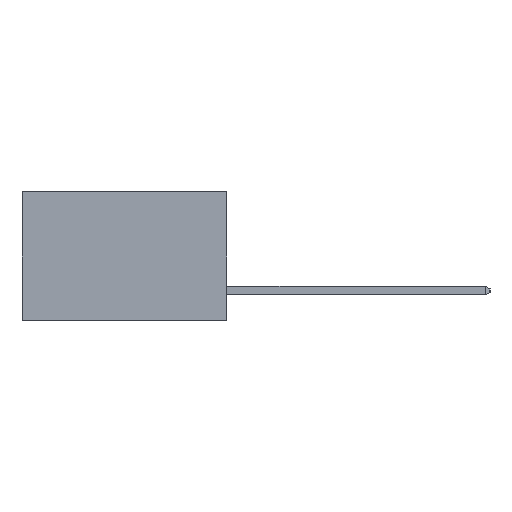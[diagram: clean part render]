
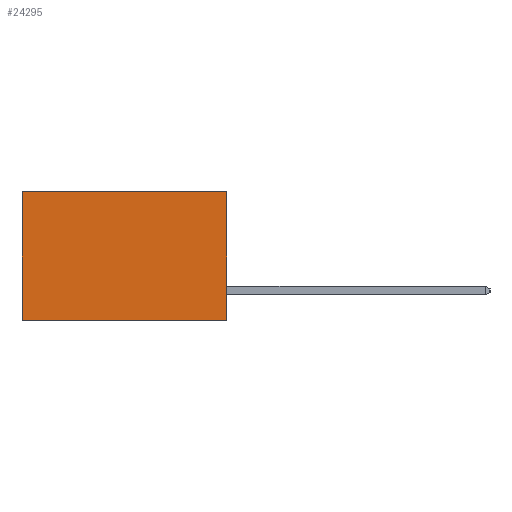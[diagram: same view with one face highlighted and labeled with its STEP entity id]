
A CAD part, left-side view. The second image highlights one B-rep face of the part: STEP entity #24295.
In plain terms, the highlighted planar face has unit normal (-1, 0, 0).
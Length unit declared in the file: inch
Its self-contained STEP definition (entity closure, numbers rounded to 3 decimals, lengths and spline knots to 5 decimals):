
#108 = FACE_OUTER_BOUND ( 'NONE', #27243, .T. ) ;
#1035 = CARTESIAN_POINT ( 'NONE',  ( 0.277, 0., -0.37 ) ) ;
#3607 = VERTEX_POINT ( 'NONE', #18103 ) ;
#3843 = VERTEX_POINT ( 'NONE', #1035 ) ;
#4120 = ORIENTED_EDGE ( 'NONE', *, *, #9924, .T. ) ;
#5090 = DIRECTION ( 'NONE',  ( 1., 0., 0. ) ) ;
#5503 = EDGE_CURVE ( 'NONE', #3607, #3843, #12586, .T. ) ;
#6590 = CARTESIAN_POINT ( 'NONE',  ( 0.277, 0.59, -0.37 ) ) ;
#7765 = CARTESIAN_POINT ( 'NONE',  ( 0.277, 0.59, 0. ) ) ;
#8504 = VERTEX_POINT ( 'NONE', #24318 ) ;
#8766 = CARTESIAN_POINT ( 'NONE',  ( 0.277, 0., -0.37 ) ) ;
#9924 = EDGE_CURVE ( 'NONE', #3607, #28241, #12692, .T. ) ;
#10095 = ORIENTED_EDGE ( 'NONE', *, *, #5503, .F. ) ;
#11259 = LINE ( 'NONE', #6590, #22120 ) ;
#11302 = DIRECTION ( 'NONE',  ( 0., 1., 0. ) ) ;
#11769 = PLANE ( 'NONE',  #25907 ) ;
#12586 = LINE ( 'NONE', #17600, #17746 ) ;
#12692 = LINE ( 'NONE', #15643, #17858 ) ;
#13662 = ORIENTED_EDGE ( 'NONE', *, *, #13940, .F. ) ;
#13713 = VECTOR ( 'NONE', #17547, 39.37008 ) ;
#13940 = EDGE_CURVE ( 'NONE', #3843, #8504, #18876, .T. ) ;
#15643 = CARTESIAN_POINT ( 'NONE',  ( 0.277, 0., 0. ) ) ;
#16268 = ORIENTED_EDGE ( 'NONE', *, *, #20449, .T. ) ;
#17547 = DIRECTION ( 'NONE',  ( 0., 1., 0. ) ) ;
#17600 = CARTESIAN_POINT ( 'NONE',  ( 0.277, 0., -0.37 ) ) ;
#17665 = DIRECTION ( 'NONE',  ( 0., 0., -1. ) ) ;
#17746 = VECTOR ( 'NONE', #17665, 39.37008 ) ;
#17754 = DIRECTION ( 'NONE',  ( 0., 0., -1. ) ) ;
#17858 = VECTOR ( 'NONE', #11302, 39.37008 ) ;
#18103 = CARTESIAN_POINT ( 'NONE',  ( 0.277, 0., 0. ) ) ;
#18418 = CARTESIAN_POINT ( 'NONE',  ( 0.277, 0., -0.37 ) ) ;
#18876 = LINE ( 'NONE', #8766, #13713 ) ;
#20449 = EDGE_CURVE ( 'NONE', #28241, #8504, #11259, .T. ) ;
#20561 = DIRECTION ( 'NONE',  ( 0., 0., -1. ) ) ;
#22120 = VECTOR ( 'NONE', #17754, 39.37008 ) ;
#24295 = ADVANCED_FACE ( 'NONE', ( #108 ), #11769, .F. ) ;
#24318 = CARTESIAN_POINT ( 'NONE',  ( 0.277, 0.59, -0.37 ) ) ;
#25907 = AXIS2_PLACEMENT_3D ( 'NONE', #18418, #5090, #20561 ) ;
#27243 = EDGE_LOOP ( 'NONE', ( #16268, #13662, #10095, #4120 ) ) ;
#28241 = VERTEX_POINT ( 'NONE', #7765 ) ;
